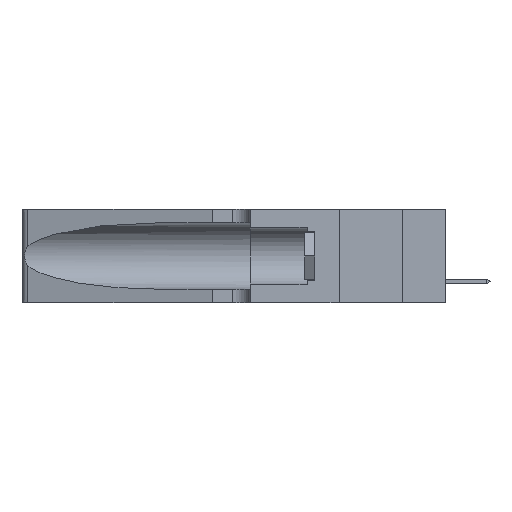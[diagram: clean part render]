
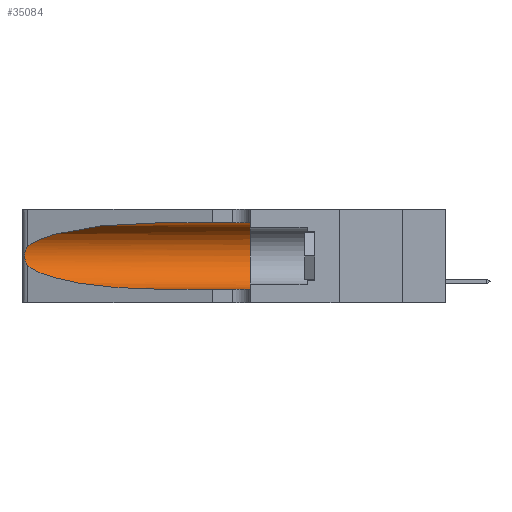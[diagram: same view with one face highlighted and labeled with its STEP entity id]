
A CAD part, left-side view. The second image highlights one B-rep face of the part: STEP entity #35084.
In plain terms, the highlighted cylindrical face has radius 3.308 mm (diameter 6.617 mm), a partial arc.
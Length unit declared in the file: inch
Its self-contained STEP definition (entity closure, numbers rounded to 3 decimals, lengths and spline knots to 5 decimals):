
#583 = EDGE_LOOP ( 'NONE', ( #34106, #5959, #44896, #46441, #36480, #30790 ) ) ;
#1656 = CARTESIAN_POINT ( 'NONE',  ( 0.25789, 1.23486, 0.15765 ) ) ;
#1968 = CARTESIAN_POINT ( 'NONE',  ( 0.18966, 0.96281, 0.31525 ) ) ;
#2205 = CARTESIAN_POINT ( 'NONE',  ( 0.1305, 1.61858, 0.31525 ) ) ;
#4475 = DIRECTION ( 'NONE',  ( 0., 0., 1. ) ) ;
#4799 = DIRECTION ( 'NONE',  ( 0., 1., 0. ) ) ;
#5959 = ORIENTED_EDGE ( 'NONE', *, *, #10508, .T. ) ;
#7420 = FACE_OUTER_BOUND ( 'NONE', #583, .T. ) ;
#8085 = VERTEX_POINT ( 'NONE', #18084 ) ;
#10508 = EDGE_CURVE ( 'NONE', #24968, #16751, #44651, .T. ) ;
#10757 = CARTESIAN_POINT ( 'NONE',  ( 0.26075, 1.23896, 0.19203 ) ) ;
#10876 = CARTESIAN_POINT ( 'NONE',  ( 0.1305, 1.61858, 0.05475 ) ) ;
#11283 = AXIS2_PLACEMENT_3D ( 'NONE', #13817, #20704, #28106 ) ;
#11309 = CARTESIAN_POINT ( 'NONE',  ( 0.25639, 1.23186, 0.15144 ) ) ;
#11719 = CIRCLE ( 'NONE', #28429, 0.13025 ) ;
#11733 = VECTOR ( 'NONE', #35852, 39.37008 ) ;
#11789 = CARTESIAN_POINT ( 'NONE',  ( 0.25487, 1.22718, 0.14631 ) ) ;
#12039 = EDGE_CURVE ( 'NONE', #22602, #24968, #42773, .T. ) ;
#12698 = CARTESIAN_POINT ( 'NONE',  ( 0.1305, 0.35, 0.05475 ) ) ;
#12974 = VECTOR ( 'NONE', #44606, 39.37008 ) ;
#13583 =( BOUNDED_CURVE ( )  B_SPLINE_CURVE ( 3, ( #11789, #14580, #33656, #37532 ),
 .UNSPECIFIED., .F., .F. ) 
 B_SPLINE_CURVE_WITH_KNOTS ( ( 4, 4 ),
 ( 3.44316, 4.71239 ),
 .UNSPECIFIED. ) 
 CURVE ( )  GEOMETRIC_REPRESENTATION_ITEM ( )  RATIONAL_B_SPLINE_CURVE ( ( 1., 0.87, 0.87, 1. ) ) 
 REPRESENTATION_ITEM ( '' )  );
#13817 = CARTESIAN_POINT ( 'NONE',  ( 0.1305, 1.61858, 0.185 ) ) ;
#14580 = CARTESIAN_POINT ( 'NONE',  ( 0.2373, 1.15595, 0.08982 ) ) ;
#15130 = CARTESIAN_POINT ( 'NONE',  ( 0.2373, 1.15595, 0.28018 ) ) ;
#15716 = EDGE_CURVE ( 'NONE', #16751, #27020, #13583, .T. ) ;
#15746 = EDGE_CURVE ( 'NONE', #27020, #37285, #45758, .T. ) ;
#16751 = VERTEX_POINT ( 'NONE', #28881 ) ;
#18084 = CARTESIAN_POINT ( 'NONE',  ( 0.1305, 0.35, 0.31525 ) ) ;
#18366 = CARTESIAN_POINT ( 'NONE',  ( 0.25487, 1.22718, 0.22369 ) ) ;
#19133 = CARTESIAN_POINT ( 'NONE',  ( 0.25555, 1.22993, 0.14849 ) ) ;
#19181 = CARTESIAN_POINT ( 'NONE',  ( 0.26075, 1.23896, 0.178 ) ) ;
#20612 = CARTESIAN_POINT ( 'NONE',  ( 0.1305, 0.72297, 0.31525 ) ) ;
#20704 = DIRECTION ( 'NONE',  ( 0., -1., 0. ) ) ;
#22602 = VERTEX_POINT ( 'NONE', #20612 ) ;
#22896 = CYLINDRICAL_SURFACE ( 'NONE', #11283, 0.13025 ) ;
#24968 = VERTEX_POINT ( 'NONE', #42880 ) ;
#26534 = CARTESIAN_POINT ( 'NONE',  ( 0.26017, 1.23833, 0.17102 ) ) ;
#27020 = VERTEX_POINT ( 'NONE', #32300 ) ;
#28106 = DIRECTION ( 'NONE',  ( 0., 0., -1. ) ) ;
#28429 = AXIS2_PLACEMENT_3D ( 'NONE', #45129, #4799, #4475 ) ;
#28881 = CARTESIAN_POINT ( 'NONE',  ( 0.25487, 1.22718, 0.14631 ) ) ;
#29607 = LINE ( 'NONE', #2205, #11733 ) ;
#30674 = CARTESIAN_POINT ( 'NONE',  ( 0.25639, 1.23184, 0.21858 ) ) ;
#30790 = ORIENTED_EDGE ( 'NONE', *, *, #42946, .F. ) ;
#32300 = CARTESIAN_POINT ( 'NONE',  ( 0.1305, 0.72297, 0.05475 ) ) ;
#33536 = CARTESIAN_POINT ( 'NONE',  ( 0.25555, 1.22994, 0.2215 ) ) ;
#33656 = CARTESIAN_POINT ( 'NONE',  ( 0.18966, 0.96281, 0.05475 ) ) ;
#34106 = ORIENTED_EDGE ( 'NONE', *, *, #12039, .T. ) ;
#34250 = CARTESIAN_POINT ( 'NONE',  ( 0.25487, 1.22718, 0.22369 ) ) ;
#34629 = CARTESIAN_POINT ( 'NONE',  ( 0.25856, 1.23593, 0.16098 ) ) ;
#35084 = ADVANCED_FACE ( 'NONE', ( #7420 ), #22896, .F. ) ;
#35852 = DIRECTION ( 'NONE',  ( 0., -1., 0. ) ) ;
#36480 = ORIENTED_EDGE ( 'NONE', *, *, #47557, .F. ) ;
#37285 = VERTEX_POINT ( 'NONE', #12698 ) ;
#37532 = CARTESIAN_POINT ( 'NONE',  ( 0.1305, 0.72297, 0.05475 ) ) ;
#38644 = CARTESIAN_POINT ( 'NONE',  ( 0.1305, 0.72297, 0.31525 ) ) ;
#38722 = CARTESIAN_POINT ( 'NONE',  ( 0.26018, 1.23835, 0.19895 ) ) ;
#40283 = CARTESIAN_POINT ( 'NONE',  ( 0.25487, 1.22718, 0.14631 ) ) ;
#42061 = CARTESIAN_POINT ( 'NONE',  ( 0.25787, 1.23484, 0.2124 ) ) ;
#42107 = CARTESIAN_POINT ( 'NONE',  ( 0.25854, 1.2359, 0.20912 ) ) ;
#42773 =( BOUNDED_CURVE ( )  B_SPLINE_CURVE ( 3, ( #38644, #1968, #15130, #34250 ),
 .UNSPECIFIED., .F., .F. ) 
 B_SPLINE_CURVE_WITH_KNOTS ( ( 4, 4 ),
 ( 1.5708, 2.84003 ),
 .UNSPECIFIED. ) 
 CURVE ( )  GEOMETRIC_REPRESENTATION_ITEM ( )  RATIONAL_B_SPLINE_CURVE ( ( 1., 0.87, 0.87, 1. ) ) 
 REPRESENTATION_ITEM ( '' )  );
#42880 = CARTESIAN_POINT ( 'NONE',  ( 0.25487, 1.22718, 0.22369 ) ) ;
#42946 = EDGE_CURVE ( 'NONE', #22602, #8085, #29607, .T. ) ;
#44606 = DIRECTION ( 'NONE',  ( 0., -1., 0. ) ) ;
#44651 = B_SPLINE_CURVE_WITH_KNOTS ( 'NONE', 3,
 ( #18366, #33536, #30674, #42061, #42107, #38722, #10757, #19181, #26534, #34629, #1656, #11309, #19133, #40283 ),
 .UNSPECIFIED., .F., .F.,
 ( 4, 2, 2, 2, 2, 2, 4 ),
 ( 0., 0.00027, 0.00053, 0.00107, 0.0016, 0.00187, 0.00214 ),
 .UNSPECIFIED. ) ;
#44896 = ORIENTED_EDGE ( 'NONE', *, *, #15716, .T. ) ;
#45129 = CARTESIAN_POINT ( 'NONE',  ( 0.1305, 0.35, 0.185 ) ) ;
#45758 = LINE ( 'NONE', #10876, #12974 ) ;
#46441 = ORIENTED_EDGE ( 'NONE', *, *, #15746, .T. ) ;
#47557 = EDGE_CURVE ( 'NONE', #8085, #37285, #11719, .T. ) ;
